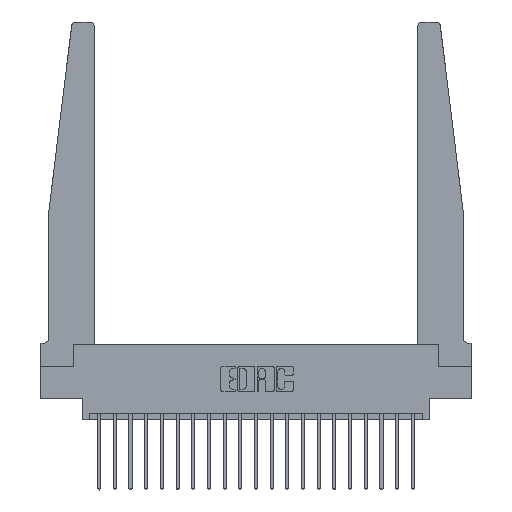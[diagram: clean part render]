
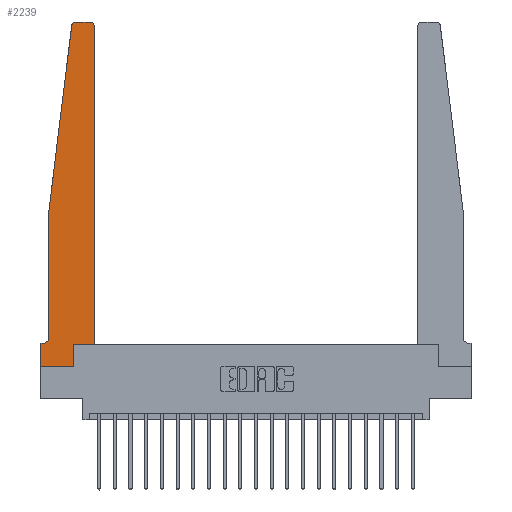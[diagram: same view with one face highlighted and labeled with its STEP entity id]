
A CAD part, top view. The second image highlights one B-rep face of the part: STEP entity #2239.
In plain terms, the highlighted planar face has unit normal (0, 0, 1).
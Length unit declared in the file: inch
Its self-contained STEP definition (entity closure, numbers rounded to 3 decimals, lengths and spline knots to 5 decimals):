
#48 = EDGE_CURVE ( 'NONE', #18803, #16221, #5648, .T. ) ;
#108 = VERTEX_POINT ( 'NONE', #18136 ) ;
#479 = DIRECTION ( 'NONE',  ( 0., 1., 0. ) ) ;
#552 = AXIS2_PLACEMENT_3D ( 'NONE', #11245, #1332, #12905 ) ;
#709 = DIRECTION ( 'NONE',  ( 0., -1., 0. ) ) ;
#760 = DIRECTION ( 'NONE',  ( -1., 0., 0. ) ) ;
#947 = DIRECTION ( 'NONE',  ( 1., 0., 0. ) ) ;
#984 = CARTESIAN_POINT ( 'NONE',  ( 0., 0., 0.37 ) ) ;
#1223 = DIRECTION ( 'NONE',  ( 1., 0., 0. ) ) ;
#1318 = ORIENTED_EDGE ( 'NONE', *, *, #48, .T. ) ;
#1332 = DIRECTION ( 'NONE',  ( 0., 0., -1. ) ) ;
#1350 = DIRECTION ( 'NONE',  ( 1., 0., 0. ) ) ;
#1532 = ORIENTED_EDGE ( 'NONE', *, *, #13242, .T. ) ;
#1567 = ORIENTED_EDGE ( 'NONE', *, *, #8595, .T. ) ;
#1594 = VERTEX_POINT ( 'NONE', #9160 ) ;
#1615 = ORIENTED_EDGE ( 'NONE', *, *, #4617, .T. ) ;
#1859 = VECTOR ( 'NONE', #11614, 39.37008 ) ;
#2239 = ADVANCED_FACE ( 'NONE', ( #18834 ), #4546, .T. ) ;
#2310 = AXIS2_PLACEMENT_3D ( 'NONE', #20818, #10871, #947 ) ;
#2393 = CARTESIAN_POINT ( 'NONE',  ( 0.065, 1.25, 0.37 ) ) ;
#2688 = EDGE_LOOP ( 'NONE', ( #1532, #15890, #12140, #1615, #14497, #18448, #5051, #11377, #3013, #11602, #1567, #1318 ) ) ;
#3013 = ORIENTED_EDGE ( 'NONE', *, *, #5175, .T. ) ;
#3586 = CARTESIAN_POINT ( 'NONE',  ( 0.2605, 0.18, 0.37 ) ) ;
#3627 = VERTEX_POINT ( 'NONE', #984 ) ;
#3819 = AXIS2_PLACEMENT_3D ( 'NONE', #19967, #19757, #19686 ) ;
#4110 = CARTESIAN_POINT ( 'NONE',  ( 0.065, 0.1875, 0.37 ) ) ;
#4546 = PLANE ( 'NONE',  #10203 ) ;
#4617 = EDGE_CURVE ( 'NONE', #108, #8374, #9009, .T. ) ;
#4802 = CARTESIAN_POINT ( 'NONE',  ( 0.25, 2.75, 0.37 ) ) ;
#4835 = VECTOR ( 'NONE', #14581, 39.37008 ) ;
#5051 = ORIENTED_EDGE ( 'NONE', *, *, #9782, .T. ) ;
#5175 = EDGE_CURVE ( 'NONE', #17835, #5662, #20695, .T. ) ;
#5533 = LINE ( 'NONE', #16116, #13828 ) ;
#5648 = CIRCLE ( 'NONE', #3819, 0.03 ) ;
#5662 = VERTEX_POINT ( 'NONE', #3586 ) ;
#6126 = EDGE_CURVE ( 'NONE', #3627, #17835, #14137, .T. ) ;
#6195 = CARTESIAN_POINT ( 'NONE',  ( 0.425, 0.18, 0.37 ) ) ;
#6245 = CARTESIAN_POINT ( 'NONE',  ( 0., 0.1875, 0.37 ) ) ;
#7248 = CARTESIAN_POINT ( 'NONE',  ( 0.065, 0.2375, 0.37 ) ) ;
#7304 = CIRCLE ( 'NONE', #552, 0.05 ) ;
#7419 = VECTOR ( 'NONE', #479, 39.37008 ) ;
#7764 = CARTESIAN_POINT ( 'NONE',  ( 0., 0., 0.37 ) ) ;
#7777 = CIRCLE ( 'NONE', #2310, 0.03 ) ;
#7889 = CARTESIAN_POINT ( 'NONE',  ( 0.065, 1.25, 0.37 ) ) ;
#8239 = CARTESIAN_POINT ( 'NONE',  ( 0., 0., 0.37 ) ) ;
#8370 = VECTOR ( 'NONE', #9838, 39.37008 ) ;
#8374 = VERTEX_POINT ( 'NONE', #7248 ) ;
#8415 = CARTESIAN_POINT ( 'NONE',  ( 0.425, 2.72, 0.37 ) ) ;
#8595 = EDGE_CURVE ( 'NONE', #9417, #18803, #5533, .T. ) ;
#8706 = CARTESIAN_POINT ( 'NONE',  ( 0.2605, 0.18, 0.37 ) ) ;
#9009 = LINE ( 'NONE', #2393, #16823 ) ;
#9160 = CARTESIAN_POINT ( 'NONE',  ( 0.27653, 2.75, 0.37 ) ) ;
#9413 = EDGE_CURVE ( 'NONE', #16156, #13406, #20812, .T. ) ;
#9417 = VERTEX_POINT ( 'NONE', #19051 ) ;
#9723 = VECTOR ( 'NONE', #1223, 39.37008 ) ;
#9782 = EDGE_CURVE ( 'NONE', #13406, #3627, #18988, .T. ) ;
#9838 = DIRECTION ( 'NONE',  ( -1., 0., 0. ) ) ;
#9903 = CARTESIAN_POINT ( 'NONE',  ( 0.015, 0.1875, 0.37 ) ) ;
#10203 = AXIS2_PLACEMENT_3D ( 'NONE', #6245, #11263, #1350 ) ;
#10660 = CARTESIAN_POINT ( 'NONE',  ( 0.2605, 0., 0.37 ) ) ;
#10871 = DIRECTION ( 'NONE',  ( 0., 0., 1. ) ) ;
#10927 = EDGE_CURVE ( 'NONE', #5662, #9417, #21233, .T. ) ;
#11245 = CARTESIAN_POINT ( 'NONE',  ( 0.015, 0.2375, 0.37 ) ) ;
#11263 = DIRECTION ( 'NONE',  ( 0., 0., 1. ) ) ;
#11377 = ORIENTED_EDGE ( 'NONE', *, *, #6126, .T. ) ;
#11602 = ORIENTED_EDGE ( 'NONE', *, *, #10927, .T. ) ;
#11614 = DIRECTION ( 'NONE',  ( 0., -1., 0. ) ) ;
#11740 = CARTESIAN_POINT ( 'NONE',  ( 0.395, 2.75, 0.37 ) ) ;
#11950 = VERTEX_POINT ( 'NONE', #21368 ) ;
#12140 = ORIENTED_EDGE ( 'NONE', *, *, #19217, .T. ) ;
#12905 = DIRECTION ( 'NONE',  ( -1., 0., 0. ) ) ;
#13104 = LINE ( 'NONE', #7889, #4835 ) ;
#13242 = EDGE_CURVE ( 'NONE', #16221, #1594, #17246, .T. ) ;
#13406 = VERTEX_POINT ( 'NONE', #15197 ) ;
#13441 = VECTOR ( 'NONE', #19514, 39.37008 ) ;
#13828 = VECTOR ( 'NONE', #17870, 39.37008 ) ;
#14137 = LINE ( 'NONE', #7764, #9723 ) ;
#14497 = ORIENTED_EDGE ( 'NONE', *, *, #21018, .T. ) ;
#14581 = DIRECTION ( 'NONE',  ( -0.122, -0.992, 0. ) ) ;
#15197 = CARTESIAN_POINT ( 'NONE',  ( 0., 0.1875, 0.37 ) ) ;
#15890 = ORIENTED_EDGE ( 'NONE', *, *, #15977, .T. ) ;
#15977 = EDGE_CURVE ( 'NONE', #1594, #11950, #7777, .T. ) ;
#16116 = CARTESIAN_POINT ( 'NONE',  ( 0.425, 0.18, 0.37 ) ) ;
#16156 = VERTEX_POINT ( 'NONE', #9903 ) ;
#16221 = VERTEX_POINT ( 'NONE', #11740 ) ;
#16389 = VECTOR ( 'NONE', #760, 39.37008 ) ;
#16823 = VECTOR ( 'NONE', #709, 39.37008 ) ;
#17246 = LINE ( 'NONE', #4802, #8370 ) ;
#17835 = VERTEX_POINT ( 'NONE', #10660 ) ;
#17870 = DIRECTION ( 'NONE',  ( 0., 1., 0. ) ) ;
#18136 = CARTESIAN_POINT ( 'NONE',  ( 0.065, 1.25, 0.37 ) ) ;
#18448 = ORIENTED_EDGE ( 'NONE', *, *, #9413, .T. ) ;
#18803 = VERTEX_POINT ( 'NONE', #8415 ) ;
#18834 = FACE_OUTER_BOUND ( 'NONE', #2688, .T. ) ;
#18988 = LINE ( 'NONE', #8239, #1859 ) ;
#19051 = CARTESIAN_POINT ( 'NONE',  ( 0.425, 0.18, 0.37 ) ) ;
#19217 = EDGE_CURVE ( 'NONE', #11950, #108, #13104, .T. ) ;
#19514 = DIRECTION ( 'NONE',  ( 1., 0., 0. ) ) ;
#19686 = DIRECTION ( 'NONE',  ( 1., 0., 0. ) ) ;
#19757 = DIRECTION ( 'NONE',  ( 0., 0., 1. ) ) ;
#19967 = CARTESIAN_POINT ( 'NONE',  ( 0.395, 2.72, 0.37 ) ) ;
#20695 = LINE ( 'NONE', #8706, #7419 ) ;
#20812 = LINE ( 'NONE', #4110, #16389 ) ;
#20818 = CARTESIAN_POINT ( 'NONE',  ( 0.27653, 2.72, 0.37 ) ) ;
#21018 = EDGE_CURVE ( 'NONE', #8374, #16156, #7304, .T. ) ;
#21233 = LINE ( 'NONE', #6195, #13441 ) ;
#21368 = CARTESIAN_POINT ( 'NONE',  ( 0.24675, 2.72367, 0.37 ) ) ;
